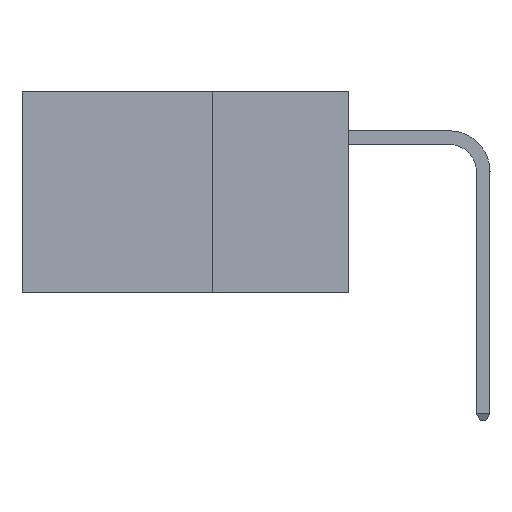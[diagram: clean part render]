
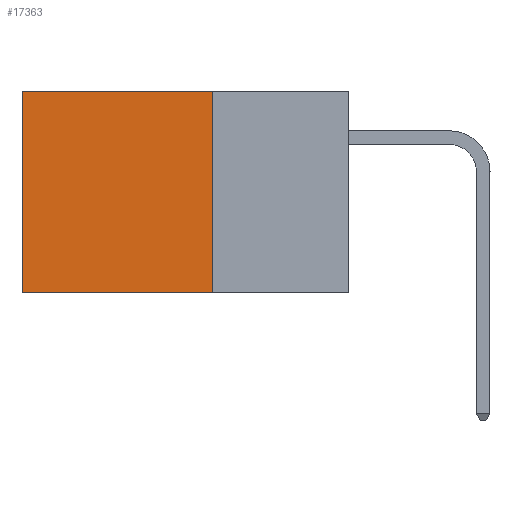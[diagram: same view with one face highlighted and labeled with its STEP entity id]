
A CAD part, left-side view. The second image highlights one B-rep face of the part: STEP entity #17363.
In plain terms, the highlighted planar face has unit normal (-1, 0, 0).
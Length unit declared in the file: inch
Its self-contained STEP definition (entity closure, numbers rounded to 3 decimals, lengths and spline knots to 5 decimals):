
#228 = VERTEX_POINT ( 'NONE', #18396 ) ;
#304 = LINE ( 'NONE', #8361, #15025 ) ;
#2381 = VECTOR ( 'NONE', #6215, 39.37008 ) ;
#2846 = DIRECTION ( 'NONE',  ( 0., 1., 0. ) ) ;
#2850 = AXIS2_PLACEMENT_3D ( 'NONE', #10617, #10283, #34252 ) ;
#2991 = EDGE_CURVE ( 'NONE', #14672, #228, #11645, .T. ) ;
#4120 = VECTOR ( 'NONE', #2846, 39.37008 ) ;
#5047 = EDGE_CURVE ( 'NONE', #23549, #14672, #29951, .T. ) ;
#5788 = ORIENTED_EDGE ( 'NONE', *, *, #26108, .F. ) ;
#6215 = DIRECTION ( 'NONE',  ( 0., 0., -1. ) ) ;
#6332 = ORIENTED_EDGE ( 'NONE', *, *, #6792, .F. ) ;
#6792 = EDGE_CURVE ( 'NONE', #25232, #228, #8957, .T. ) ;
#7001 = CARTESIAN_POINT ( 'NONE',  ( 0.2875, 0.25, 0. ) ) ;
#8361 = CARTESIAN_POINT ( 'NONE',  ( 0.2875, 0.25, 0. ) ) ;
#8957 = LINE ( 'NONE', #19626, #4120 ) ;
#10283 = DIRECTION ( 'NONE',  ( 1., 0., 0. ) ) ;
#10617 = CARTESIAN_POINT ( 'NONE',  ( 0.2875, 0.25, 0. ) ) ;
#10986 = DIRECTION ( 'NONE',  ( 0., 0., -1. ) ) ;
#11645 = LINE ( 'NONE', #28106, #2381 ) ;
#14377 = CARTESIAN_POINT ( 'NONE',  ( 0.2875, 0.25, 0. ) ) ;
#14672 = VERTEX_POINT ( 'NONE', #16742 ) ;
#15025 = VECTOR ( 'NONE', #10986, 39.37008 ) ;
#16742 = CARTESIAN_POINT ( 'NONE',  ( 0.2875, 0.6, 0. ) ) ;
#17363 = ADVANCED_FACE ( 'NONE', ( #29353 ), #26720, .F. ) ;
#18396 = CARTESIAN_POINT ( 'NONE',  ( 0.2875, 0.6, -0.37 ) ) ;
#19442 = DIRECTION ( 'NONE',  ( 0., 1., 0. ) ) ;
#19626 = CARTESIAN_POINT ( 'NONE',  ( 0.2875, 0.25, -0.37 ) ) ;
#23549 = VERTEX_POINT ( 'NONE', #7001 ) ;
#25232 = VERTEX_POINT ( 'NONE', #28984 ) ;
#26108 = EDGE_CURVE ( 'NONE', #23549, #25232, #304, .T. ) ;
#26295 = VECTOR ( 'NONE', #19442, 39.37008 ) ;
#26720 = PLANE ( 'NONE',  #2850 ) ;
#27112 = ORIENTED_EDGE ( 'NONE', *, *, #2991, .T. ) ;
#27556 = EDGE_LOOP ( 'NONE', ( #27112, #6332, #5788, #29417 ) ) ;
#28106 = CARTESIAN_POINT ( 'NONE',  ( 0.2875, 0.6, 0. ) ) ;
#28984 = CARTESIAN_POINT ( 'NONE',  ( 0.2875, 0.25, -0.37 ) ) ;
#29353 = FACE_OUTER_BOUND ( 'NONE', #27556, .T. ) ;
#29417 = ORIENTED_EDGE ( 'NONE', *, *, #5047, .T. ) ;
#29951 = LINE ( 'NONE', #14377, #26295 ) ;
#34252 = DIRECTION ( 'NONE',  ( 0., 0., -1. ) ) ;
